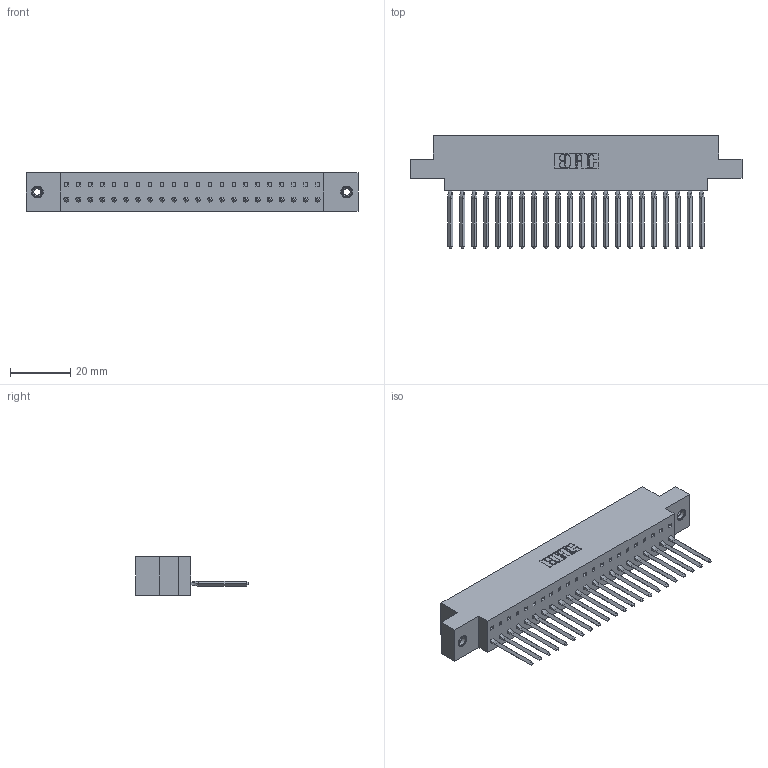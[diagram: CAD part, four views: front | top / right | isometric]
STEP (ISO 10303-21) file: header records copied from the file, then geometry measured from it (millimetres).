
FILE_DESCRIPTION (( 'STEP AP203' ), '1' );
FILE_NAME ('317-022-541-608.STEP', '2020-02-27T17:18:51', ( '' ), ( '' ), 'SwSTEP 2.0', 'SolidWorks 2016', '' );
FILE_SCHEMA (( 'CONFIG_CONTROL_DESIGN' ));
Length unit declared in the file: inch
Products named in the file (4): 317-290-002_541; 345-250-001_345-250-003-102; 317-022-541-608; 317 Part_.156 Dia - TI
Assembly tree (25 placements, depth 2):
  317-022-541-608
    317 Part_.156 Dia - TI
    317-290-002_541  x22
    345-250-001_345-250-003-102  x2
Bounding box: 109.88 x 37.34 x 12.7 mm (x, y, z)
Volume: 17197.4 mm3; surface area: 23655.9 mm2
Topology: 25 solids, 25 shells, 3506 faces, 9959 edges, 6470 vertices
Faces by surface type: plane 2818, cylinder 584, bspline 88, cone 12, torus 4
Entity records: 36621 total; most frequent: CARTESIAN_POINT 7110, ORIENTED_EDGE 6378, DIRECTION 5267, EDGE_CURVE 3189, LINE 2805, VECTOR 2805, VERTEX_POINT 2114, AXIS2_PLACEMENT_3D 1231
